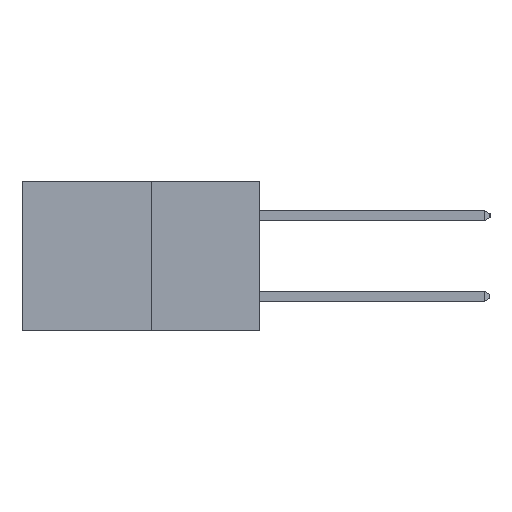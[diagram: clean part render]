
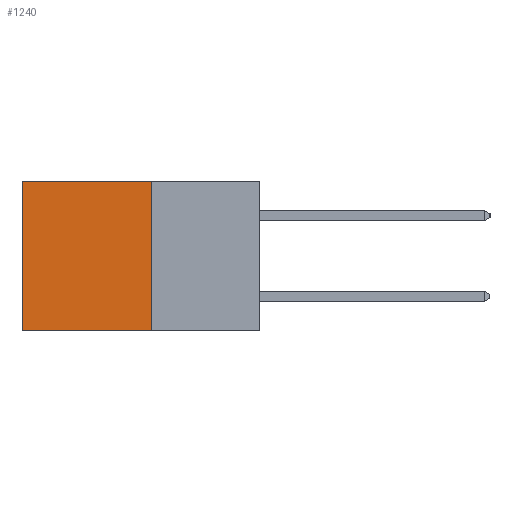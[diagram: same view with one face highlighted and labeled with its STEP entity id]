
A CAD part, left-side view. The second image highlights one B-rep face of the part: STEP entity #1240.
In plain terms, the highlighted planar face has unit normal (-1, 0, 0).
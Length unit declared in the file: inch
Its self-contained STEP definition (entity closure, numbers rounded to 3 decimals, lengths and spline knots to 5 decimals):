
#29 = EDGE_CURVE ( 'NONE', #10870, #11043, #8204, .T. ) ;
#37 = DIRECTION ( 'NONE',  ( 0., 0., -1. ) ) ;
#380 = VERTEX_POINT ( 'NONE', #2517 ) ;
#431 = CARTESIAN_POINT ( 'NONE',  ( 0.277, 0.27, 0. ) ) ;
#1009 = FACE_OUTER_BOUND ( 'NONE', #11607, .T. ) ;
#1240 = ADVANCED_FACE ( 'NONE', ( #1009 ), #1676, .F. ) ;
#1676 = PLANE ( 'NONE',  #8322 ) ;
#1708 = DIRECTION ( 'NONE',  ( 1., 0., 0. ) ) ;
#2517 = CARTESIAN_POINT ( 'NONE',  ( 0.277, 0.59, -0.37 ) ) ;
#4058 = DIRECTION ( 'NONE',  ( 0., 1., 0. ) ) ;
#4643 = ORIENTED_EDGE ( 'NONE', *, *, #29, .T. ) ;
#4987 = EDGE_CURVE ( 'NONE', #11043, #380, #13005, .T. ) ;
#5295 = LINE ( 'NONE', #8474, #10068 ) ;
#6941 = DIRECTION ( 'NONE',  ( 0., 1., 0. ) ) ;
#6999 = VECTOR ( 'NONE', #11279, 39.37008 ) ;
#7728 = VECTOR ( 'NONE', #4058, 39.37008 ) ;
#7736 = CARTESIAN_POINT ( 'NONE',  ( 0.277, 0.27, -0.37 ) ) ;
#7782 = CARTESIAN_POINT ( 'NONE',  ( 0.277, 0.27, 0. ) ) ;
#8204 = LINE ( 'NONE', #7782, #13506 ) ;
#8322 = AXIS2_PLACEMENT_3D ( 'NONE', #7736, #1708, #37 ) ;
#8474 = CARTESIAN_POINT ( 'NONE',  ( 0.277, 0.27, -0.37 ) ) ;
#8521 = CARTESIAN_POINT ( 'NONE',  ( 0.277, 0.27, -0.37 ) ) ;
#9487 = ORIENTED_EDGE ( 'NONE', *, *, #4987, .T. ) ;
#9547 = DIRECTION ( 'NONE',  ( 0., 0., -1. ) ) ;
#9760 = EDGE_CURVE ( 'NONE', #10870, #11218, #5295, .T. ) ;
#10068 = VECTOR ( 'NONE', #9547, 39.37008 ) ;
#10701 = ORIENTED_EDGE ( 'NONE', *, *, #11709, .F. ) ;
#10870 = VERTEX_POINT ( 'NONE', #431 ) ;
#10897 = CARTESIAN_POINT ( 'NONE',  ( 0.277, 0.27, -0.37 ) ) ;
#11043 = VERTEX_POINT ( 'NONE', #12766 ) ;
#11218 = VERTEX_POINT ( 'NONE', #10897 ) ;
#11279 = DIRECTION ( 'NONE',  ( 0., 0., -1. ) ) ;
#11607 = EDGE_LOOP ( 'NONE', ( #9487, #10701, #12584, #4643 ) ) ;
#11694 = CARTESIAN_POINT ( 'NONE',  ( 0.277, 0.59, -0.37 ) ) ;
#11709 = EDGE_CURVE ( 'NONE', #11218, #380, #13054, .T. ) ;
#12584 = ORIENTED_EDGE ( 'NONE', *, *, #9760, .F. ) ;
#12766 = CARTESIAN_POINT ( 'NONE',  ( 0.277, 0.59, 0. ) ) ;
#13005 = LINE ( 'NONE', #11694, #6999 ) ;
#13054 = LINE ( 'NONE', #8521, #7728 ) ;
#13506 = VECTOR ( 'NONE', #6941, 39.37008 ) ;
